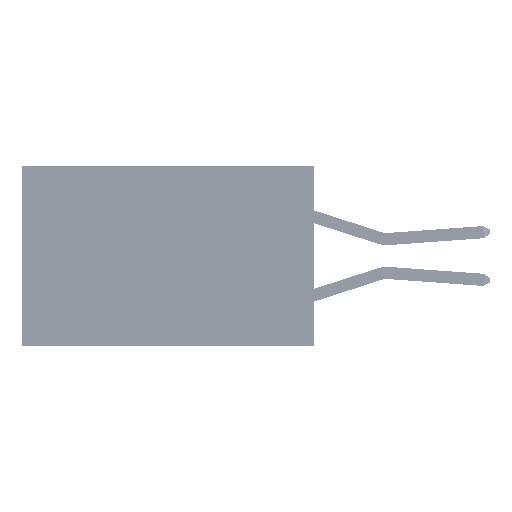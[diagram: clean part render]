
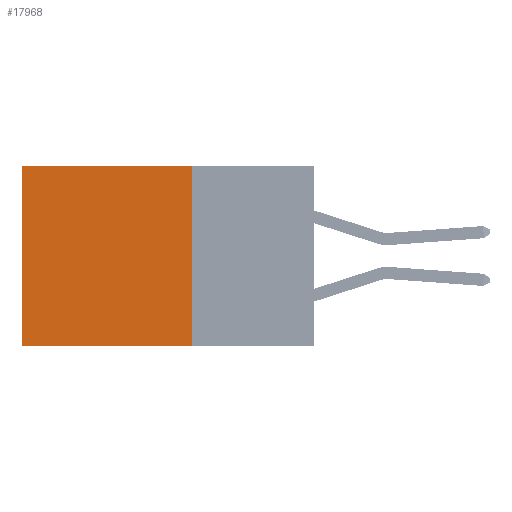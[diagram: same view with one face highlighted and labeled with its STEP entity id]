
A CAD part, left-side view. The second image highlights one B-rep face of the part: STEP entity #17968.
In plain terms, the highlighted planar face has unit normal (-1, 0, 0).
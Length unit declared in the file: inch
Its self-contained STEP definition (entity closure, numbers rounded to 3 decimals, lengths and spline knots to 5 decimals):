
#2433 = VERTEX_POINT ( 'NONE', #7855 ) ;
#2437 = ORIENTED_EDGE ( 'NONE', *, *, #43885, .F. ) ;
#4586 = VECTOR ( 'NONE', #6927, 39.37008 ) ;
#5249 = ORIENTED_EDGE ( 'NONE', *, *, #12354, .T. ) ;
#6584 = ORIENTED_EDGE ( 'NONE', *, *, #41110, .F. ) ;
#6757 = FACE_OUTER_BOUND ( 'NONE', #34991, .T. ) ;
#6927 = DIRECTION ( 'NONE',  ( 0., 1., 0. ) ) ;
#7378 = VERTEX_POINT ( 'NONE', #32328 ) ;
#7768 = DIRECTION ( 'NONE',  ( 0., 0., -1. ) ) ;
#7799 = LINE ( 'NONE', #17652, #28678 ) ;
#7855 = CARTESIAN_POINT ( 'NONE',  ( 0.2875, 0.6, 0. ) ) ;
#12354 = EDGE_CURVE ( 'NONE', #2433, #7378, #7799, .T. ) ;
#16785 = DIRECTION ( 'NONE',  ( 0., 1., 0. ) ) ;
#17652 = CARTESIAN_POINT ( 'NONE',  ( 0.2875, 0.6, 0. ) ) ;
#17968 = ADVANCED_FACE ( 'NONE', ( #6757 ), #27969, .F. ) ;
#18166 = VERTEX_POINT ( 'NONE', #25791 ) ;
#19466 = LINE ( 'NONE', #30471, #45711 ) ;
#23981 = CARTESIAN_POINT ( 'NONE',  ( 0.2875, 0.25, 0. ) ) ;
#24310 = DIRECTION ( 'NONE',  ( 1., 0., 0. ) ) ;
#25791 = CARTESIAN_POINT ( 'NONE',  ( 0.2875, 0.25, -0.37 ) ) ;
#27969 = PLANE ( 'NONE',  #35758 ) ;
#28678 = VECTOR ( 'NONE', #32834, 39.37008 ) ;
#29694 = LINE ( 'NONE', #35978, #33261 ) ;
#30275 = LINE ( 'NONE', #44747, #4586 ) ;
#30471 = CARTESIAN_POINT ( 'NONE',  ( 0.2875, 0.25, 0. ) ) ;
#32328 = CARTESIAN_POINT ( 'NONE',  ( 0.2875, 0.6, -0.37 ) ) ;
#32834 = DIRECTION ( 'NONE',  ( 0., 0., -1. ) ) ;
#33261 = VECTOR ( 'NONE', #16785, 39.37008 ) ;
#34991 = EDGE_LOOP ( 'NONE', ( #5249, #6584, #2437, #37861 ) ) ;
#35758 = AXIS2_PLACEMENT_3D ( 'NONE', #23981, #24310, #42936 ) ;
#35978 = CARTESIAN_POINT ( 'NONE',  ( 0.2875, 0.25, 0. ) ) ;
#37861 = ORIENTED_EDGE ( 'NONE', *, *, #40908, .T. ) ;
#40908 = EDGE_CURVE ( 'NONE', #44297, #2433, #29694, .T. ) ;
#41110 = EDGE_CURVE ( 'NONE', #18166, #7378, #30275, .T. ) ;
#42936 = DIRECTION ( 'NONE',  ( 0., 0., -1. ) ) ;
#43229 = CARTESIAN_POINT ( 'NONE',  ( 0.2875, 0.25, 0. ) ) ;
#43885 = EDGE_CURVE ( 'NONE', #44297, #18166, #19466, .T. ) ;
#44297 = VERTEX_POINT ( 'NONE', #43229 ) ;
#44747 = CARTESIAN_POINT ( 'NONE',  ( 0.2875, 0.25, -0.37 ) ) ;
#45711 = VECTOR ( 'NONE', #7768, 39.37008 ) ;
